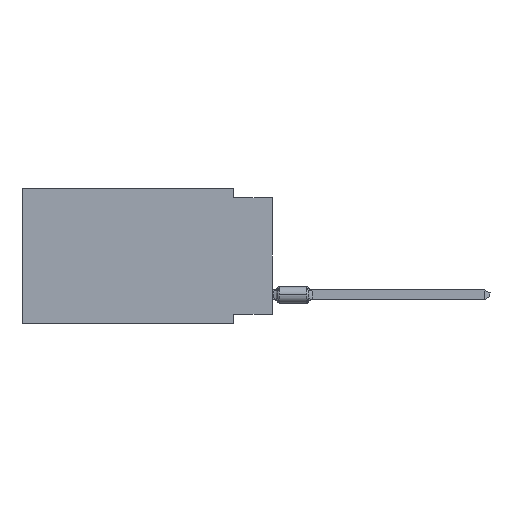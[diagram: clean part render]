
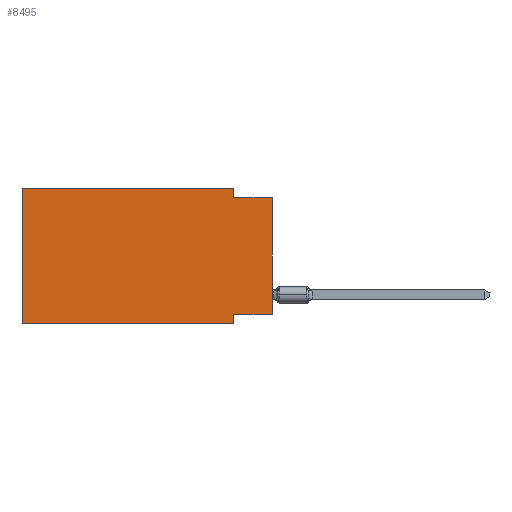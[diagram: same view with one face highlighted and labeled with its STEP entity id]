
A CAD part, left-side view. The second image highlights one B-rep face of the part: STEP entity #8495.
In plain terms, the highlighted planar face has unit normal (-1, 0, 0).
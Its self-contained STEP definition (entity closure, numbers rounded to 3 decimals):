
#210 = EDGE_LOOP ( 'NONE', ( #18390, #32298, #23833, #36537, #36670, #35559, #21948, #811 ) ) ;
#811 = ORIENTED_EDGE ( 'NONE', *, *, #39821, .F. ) ;
#1276 = LINE ( 'NONE', #8253, #36364 ) ;
#1382 = LINE ( 'NONE', #29913, #35145 ) ;
#3971 = LINE ( 'NONE', #28807, #35677 ) ;
#4280 = DIRECTION ( 'NONE',  ( 1., 0., 0. ) ) ;
#4285 = DIRECTION ( 'NONE',  ( 0., 0., -1. ) ) ;
#4494 = VERTEX_POINT ( 'NONE', #5338 ) ;
#5338 = CARTESIAN_POINT ( 'NONE',  ( 0., 2.54, -8.255 ) ) ;
#6547 = DIRECTION ( 'NONE',  ( 0., -1., 0. ) ) ;
#7140 = CARTESIAN_POINT ( 'NONE',  ( 0., 16.383, -8.89 ) ) ;
#7725 = EDGE_CURVE ( 'NONE', #4494, #15614, #1382, .T. ) ;
#8253 = CARTESIAN_POINT ( 'NONE',  ( 0., 16.383, 0. ) ) ;
#8437 = VECTOR ( 'NONE', #34393, 1000. ) ;
#8495 = ADVANCED_FACE ( 'NONE', ( #35673 ), #16997, .F. ) ;
#8634 = CARTESIAN_POINT ( 'NONE',  ( 0., 16.383, 0. ) ) ;
#8957 = LINE ( 'NONE', #27625, #9826 ) ;
#9203 = CARTESIAN_POINT ( 'NONE',  ( 0., 16.383, -8.89 ) ) ;
#9826 = VECTOR ( 'NONE', #30888, 1000. ) ;
#10571 = LINE ( 'NONE', #9203, #21813 ) ;
#13716 = VECTOR ( 'NONE', #40221, 1000. ) ;
#15614 = VERTEX_POINT ( 'NONE', #24921 ) ;
#16330 = CARTESIAN_POINT ( 'NONE',  ( 0., 0., 0. ) ) ;
#16997 = PLANE ( 'NONE',  #25090 ) ;
#18390 = ORIENTED_EDGE ( 'NONE', *, *, #32719, .T. ) ;
#18742 = CARTESIAN_POINT ( 'NONE',  ( 0., 2.54, 0. ) ) ;
#19466 = EDGE_CURVE ( 'NONE', #21900, #19947, #1276, .T. ) ;
#19947 = VERTEX_POINT ( 'NONE', #18742 ) ;
#20777 = DIRECTION ( 'NONE',  ( 0., -1., 0. ) ) ;
#21813 = VECTOR ( 'NONE', #6547, 1000. ) ;
#21868 = LINE ( 'NONE', #16330, #8437 ) ;
#21900 = VERTEX_POINT ( 'NONE', #33605 ) ;
#21948 = ORIENTED_EDGE ( 'NONE', *, *, #7725, .F. ) ;
#22800 = EDGE_CURVE ( 'NONE', #23492, #21900, #30786, .T. ) ;
#22925 = CARTESIAN_POINT ( 'NONE',  ( 0., 0., -8.255 ) ) ;
#23039 = DIRECTION ( 'NONE',  ( 0., -1., 0. ) ) ;
#23492 = VERTEX_POINT ( 'NONE', #7140 ) ;
#23833 = ORIENTED_EDGE ( 'NONE', *, *, #33793, .F. ) ;
#24921 = CARTESIAN_POINT ( 'NONE',  ( 0., 2.54, -8.89 ) ) ;
#24950 = VERTEX_POINT ( 'NONE', #22925 ) ;
#24958 = DIRECTION ( 'NONE',  ( 0., 1., 0. ) ) ;
#25090 = AXIS2_PLACEMENT_3D ( 'NONE', #29113, #4280, #36081 ) ;
#25948 = CARTESIAN_POINT ( 'NONE',  ( 0., 0., -0.635 ) ) ;
#27490 = VERTEX_POINT ( 'NONE', #25948 ) ;
#27625 = CARTESIAN_POINT ( 'NONE',  ( 0., 2.54, 0. ) ) ;
#28807 = CARTESIAN_POINT ( 'NONE',  ( 0., 0., -0.635 ) ) ;
#29113 = CARTESIAN_POINT ( 'NONE',  ( 0., 16.383, 0. ) ) ;
#29913 = CARTESIAN_POINT ( 'NONE',  ( 0., 2.54, -8.89 ) ) ;
#30606 = VERTEX_POINT ( 'NONE', #35425 ) ;
#30786 = LINE ( 'NONE', #8634, #13716 ) ;
#30888 = DIRECTION ( 'NONE',  ( 0., 0., -1. ) ) ;
#32298 = ORIENTED_EDGE ( 'NONE', *, *, #40280, .F. ) ;
#32719 = EDGE_CURVE ( 'NONE', #24950, #27490, #21868, .T. ) ;
#33605 = CARTESIAN_POINT ( 'NONE',  ( 0., 16.383, 0. ) ) ;
#33676 = VECTOR ( 'NONE', #24958, 1000. ) ;
#33793 = EDGE_CURVE ( 'NONE', #19947, #30606, #8957, .T. ) ;
#34393 = DIRECTION ( 'NONE',  ( 0., 0., 1. ) ) ;
#35145 = VECTOR ( 'NONE', #4285, 1000. ) ;
#35425 = CARTESIAN_POINT ( 'NONE',  ( 0., 2.54, -0.635 ) ) ;
#35559 = ORIENTED_EDGE ( 'NONE', *, *, #38709, .T. ) ;
#35673 = FACE_OUTER_BOUND ( 'NONE', #210, .T. ) ;
#35677 = VECTOR ( 'NONE', #23039, 1000. ) ;
#36081 = DIRECTION ( 'NONE',  ( 0., 0., -1. ) ) ;
#36364 = VECTOR ( 'NONE', #20777, 1000. ) ;
#36537 = ORIENTED_EDGE ( 'NONE', *, *, #19466, .F. ) ;
#36670 = ORIENTED_EDGE ( 'NONE', *, *, #22800, .F. ) ;
#37685 = LINE ( 'NONE', #40547, #33676 ) ;
#38709 = EDGE_CURVE ( 'NONE', #23492, #15614, #10571, .T. ) ;
#39821 = EDGE_CURVE ( 'NONE', #24950, #4494, #37685, .T. ) ;
#40221 = DIRECTION ( 'NONE',  ( 0., 0., 1. ) ) ;
#40280 = EDGE_CURVE ( 'NONE', #30606, #27490, #3971, .T. ) ;
#40547 = CARTESIAN_POINT ( 'NONE',  ( 0., 0., -8.255 ) ) ;
